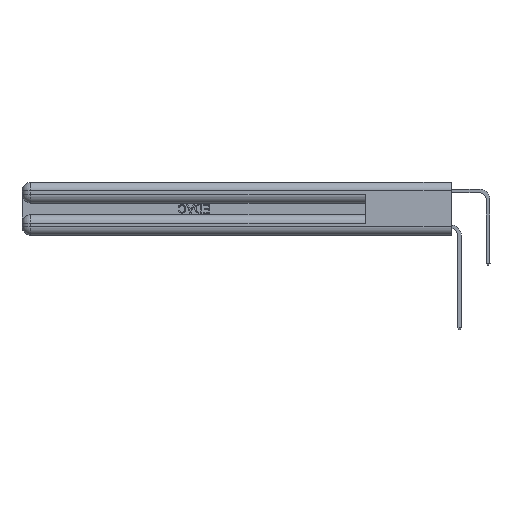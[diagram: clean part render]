
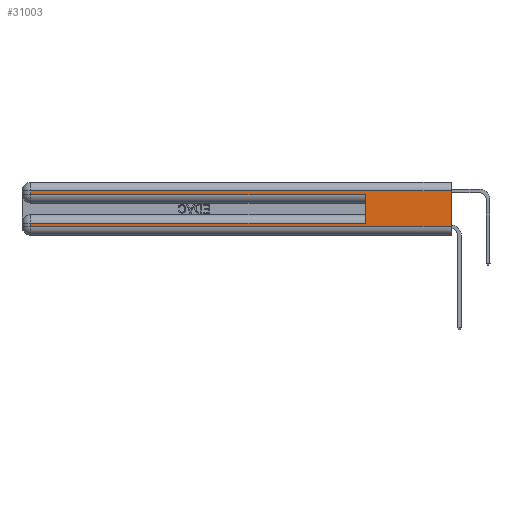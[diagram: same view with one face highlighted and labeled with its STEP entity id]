
A CAD part, left-side view. The second image highlights one B-rep face of the part: STEP entity #31003.
In plain terms, the highlighted planar face has unit normal (-1, 0, 0).
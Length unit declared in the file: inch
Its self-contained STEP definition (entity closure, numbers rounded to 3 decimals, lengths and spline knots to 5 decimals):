
#336 = ORIENTED_EDGE ( 'NONE', *, *, #18757, .T. ) ;
#602 = VECTOR ( 'NONE', #5897, 39.37008 ) ;
#1030 = CARTESIAN_POINT ( 'NONE',  ( 0., 2.94, 0.37 ) ) ;
#1225 = EDGE_CURVE ( 'NONE', #23654, #7969, #18406, .T. ) ;
#1259 = ORIENTED_EDGE ( 'NONE', *, *, #31170, .F. ) ;
#3309 = EDGE_LOOP ( 'NONE', ( #1259, #336, #19955, #7004, #19239, #5280, #4628, #14297 ) ) ;
#3505 = CARTESIAN_POINT ( 'NONE',  ( 0., 0., 0.37 ) ) ;
#3754 = EDGE_CURVE ( 'NONE', #8786, #8874, #31416, .T. ) ;
#3761 = CARTESIAN_POINT ( 'NONE',  ( 0., 2.94, 0.31 ) ) ;
#4628 = ORIENTED_EDGE ( 'NONE', *, *, #32695, .T. ) ;
#4941 = VECTOR ( 'NONE', #20997, 39.37008 ) ;
#4999 = DIRECTION ( 'NONE',  ( 0., 0., -1. ) ) ;
#5280 = ORIENTED_EDGE ( 'NONE', *, *, #1225, .T. ) ;
#5358 = DIRECTION ( 'NONE',  ( 1., 0., 0. ) ) ;
#5897 = DIRECTION ( 'NONE',  ( 0., 0., 1. ) ) ;
#6067 = VECTOR ( 'NONE', #27128, 39.37008 ) ;
#6477 = LINE ( 'NONE', #31894, #26855 ) ;
#7004 = ORIENTED_EDGE ( 'NONE', *, *, #3754, .T. ) ;
#7969 = VERTEX_POINT ( 'NONE', #23483 ) ;
#8055 = CARTESIAN_POINT ( 'NONE',  ( 0., 0., 0.31 ) ) ;
#8254 = AXIS2_PLACEMENT_3D ( 'NONE', #13267, #5358, #22877 ) ;
#8663 = DIRECTION ( 'NONE',  ( 0., 1., 0. ) ) ;
#8786 = VERTEX_POINT ( 'NONE', #15830 ) ;
#8874 = VERTEX_POINT ( 'NONE', #23914 ) ;
#10652 = CARTESIAN_POINT ( 'NONE',  ( 0., 0., 0.085 ) ) ;
#11082 = DIRECTION ( 'NONE',  ( 0., 0., -1. ) ) ;
#11445 = CARTESIAN_POINT ( 'NONE',  ( 0., 0.6, 0.145 ) ) ;
#11960 = VERTEX_POINT ( 'NONE', #3761 ) ;
#13267 = CARTESIAN_POINT ( 'NONE',  ( 0., 0., 0.37 ) ) ;
#13663 = CARTESIAN_POINT ( 'NONE',  ( 0., 2.94, 0.06 ) ) ;
#13741 = LINE ( 'NONE', #31926, #4941 ) ;
#14297 = ORIENTED_EDGE ( 'NONE', *, *, #29344, .T. ) ;
#15830 = CARTESIAN_POINT ( 'NONE',  ( 0., 2.94, 0.285 ) ) ;
#16538 = LINE ( 'NONE', #1030, #6067 ) ;
#18239 = DIRECTION ( 'NONE',  ( 0., 1., 0. ) ) ;
#18406 = LINE ( 'NONE', #10652, #24300 ) ;
#18465 = CARTESIAN_POINT ( 'NONE',  ( 0., 0., 0.285 ) ) ;
#18757 = EDGE_CURVE ( 'NONE', #25171, #11960, #6477, .T. ) ;
#19005 = LINE ( 'NONE', #3505, #21177 ) ;
#19239 = ORIENTED_EDGE ( 'NONE', *, *, #20990, .F. ) ;
#19955 = ORIENTED_EDGE ( 'NONE', *, *, #30214, .T. ) ;
#20990 = EDGE_CURVE ( 'NONE', #23654, #8874, #23755, .T. ) ;
#20997 = DIRECTION ( 'NONE',  ( 0., -1., 0. ) ) ;
#21177 = VECTOR ( 'NONE', #11082, 39.37008 ) ;
#22232 = VECTOR ( 'NONE', #4999, 39.37008 ) ;
#22877 = DIRECTION ( 'NONE',  ( 0., 0., -1. ) ) ;
#23180 = LINE ( 'NONE', #28215, #22232 ) ;
#23483 = CARTESIAN_POINT ( 'NONE',  ( 0., 2.94, 0.085 ) ) ;
#23654 = VERTEX_POINT ( 'NONE', #31995 ) ;
#23755 = LINE ( 'NONE', #11445, #602 ) ;
#23914 = CARTESIAN_POINT ( 'NONE',  ( 0., 0.6, 0.285 ) ) ;
#24300 = VECTOR ( 'NONE', #18239, 39.37008 ) ;
#25171 = VERTEX_POINT ( 'NONE', #8055 ) ;
#25879 = DIRECTION ( 'NONE',  ( 0., -1., 0. ) ) ;
#26855 = VECTOR ( 'NONE', #8663, 39.37008 ) ;
#27128 = DIRECTION ( 'NONE',  ( 0., 0., -1. ) ) ;
#28215 = CARTESIAN_POINT ( 'NONE',  ( 0., 2.94, 0.37 ) ) ;
#29344 = EDGE_CURVE ( 'NONE', #31897, #30195, #13741, .T. ) ;
#30195 = VERTEX_POINT ( 'NONE', #32188 ) ;
#30214 = EDGE_CURVE ( 'NONE', #11960, #8786, #16538, .T. ) ;
#30447 = FACE_OUTER_BOUND ( 'NONE', #3309, .T. ) ;
#31003 = ADVANCED_FACE ( 'NONE', ( #30447 ), #31115, .F. ) ;
#31115 = PLANE ( 'NONE',  #8254 ) ;
#31170 = EDGE_CURVE ( 'NONE', #25171, #30195, #19005, .T. ) ;
#31416 = LINE ( 'NONE', #18465, #31993 ) ;
#31894 = CARTESIAN_POINT ( 'NONE',  ( 0., 0., 0.31 ) ) ;
#31897 = VERTEX_POINT ( 'NONE', #13663 ) ;
#31926 = CARTESIAN_POINT ( 'NONE',  ( 0., 0., 0.06 ) ) ;
#31993 = VECTOR ( 'NONE', #25879, 39.37008 ) ;
#31995 = CARTESIAN_POINT ( 'NONE',  ( 0., 0.6, 0.085 ) ) ;
#32188 = CARTESIAN_POINT ( 'NONE',  ( 0., 0., 0.06 ) ) ;
#32695 = EDGE_CURVE ( 'NONE', #7969, #31897, #23180, .T. ) ;
